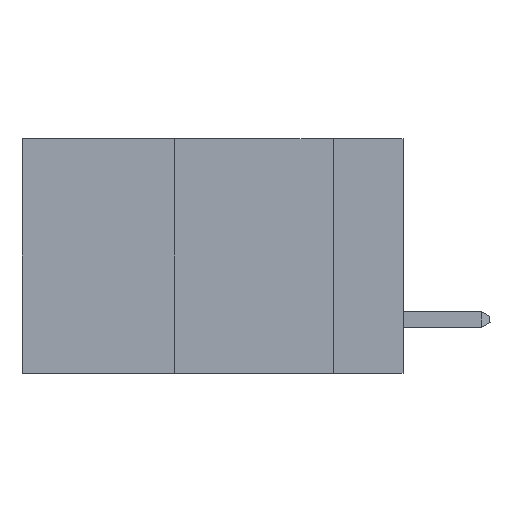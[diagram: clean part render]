
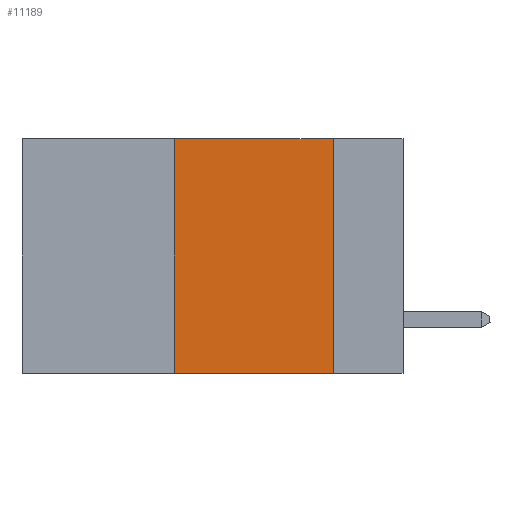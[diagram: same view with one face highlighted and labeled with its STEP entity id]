
A CAD part, left-side view. The second image highlights one B-rep face of the part: STEP entity #11189.
In plain terms, the highlighted planar face has unit normal (-1, 0, 0).
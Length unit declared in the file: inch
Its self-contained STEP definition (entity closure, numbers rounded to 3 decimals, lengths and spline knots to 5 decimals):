
#518 = VECTOR ( 'NONE', #11924, 39.37008 ) ;
#676 = ORIENTED_EDGE ( 'NONE', *, *, #15945, .F. ) ;
#3219 = DIRECTION ( 'NONE',  ( 0., 0., 1. ) ) ;
#4948 = VERTEX_POINT ( 'NONE', #10460 ) ;
#5170 = CARTESIAN_POINT ( 'NONE',  ( 0., 0.36, 0. ) ) ;
#6214 = CARTESIAN_POINT ( 'NONE',  ( 0., 0.6, 0. ) ) ;
#6275 = PLANE ( 'NONE',  #13305 ) ;
#6618 = VECTOR ( 'NONE', #9168, 39.37008 ) ;
#7361 = CARTESIAN_POINT ( 'NONE',  ( 0., 0.11, 0. ) ) ;
#7703 = DIRECTION ( 'NONE',  ( 0., 0., -1. ) ) ;
#7907 = ORIENTED_EDGE ( 'NONE', *, *, #16621, .F. ) ;
#9168 = DIRECTION ( 'NONE',  ( 0., -1., 0. ) ) ;
#9289 = VECTOR ( 'NONE', #3219, 39.37008 ) ;
#10460 = CARTESIAN_POINT ( 'NONE',  ( 0., 0.11, -0.37 ) ) ;
#11070 = ORIENTED_EDGE ( 'NONE', *, *, #15046, .F. ) ;
#11098 = LINE ( 'NONE', #15953, #6618 ) ;
#11189 = ADVANCED_FACE ( 'NONE', ( #14646 ), #6275, .F. ) ;
#11464 = DIRECTION ( 'NONE',  ( 0., 0., -1. ) ) ;
#11812 = LINE ( 'NONE', #14694, #518 ) ;
#11924 = DIRECTION ( 'NONE',  ( 0., -1., 0. ) ) ;
#13004 = VERTEX_POINT ( 'NONE', #16023 ) ;
#13062 = CARTESIAN_POINT ( 'NONE',  ( 0., 0.36, 0. ) ) ;
#13305 = AXIS2_PLACEMENT_3D ( 'NONE', #6214, #15879, #7703 ) ;
#13361 = VECTOR ( 'NONE', #11464, 39.37008 ) ;
#13809 = LINE ( 'NONE', #7361, #13361 ) ;
#14348 = EDGE_LOOP ( 'NONE', ( #11070, #7907, #676, #15606 ) ) ;
#14646 = FACE_OUTER_BOUND ( 'NONE', #14348, .T. ) ;
#14694 = CARTESIAN_POINT ( 'NONE',  ( 0., 0.6, 0. ) ) ;
#14949 = VERTEX_POINT ( 'NONE', #16719 ) ;
#15046 = EDGE_CURVE ( 'NONE', #14949, #4948, #13809, .T. ) ;
#15606 = ORIENTED_EDGE ( 'NONE', *, *, #17745, .T. ) ;
#15879 = DIRECTION ( 'NONE',  ( 1., 0., 0. ) ) ;
#15945 = EDGE_CURVE ( 'NONE', #13004, #16123, #16526, .T. ) ;
#15953 = CARTESIAN_POINT ( 'NONE',  ( 0., 0.6, -0.37 ) ) ;
#16023 = CARTESIAN_POINT ( 'NONE',  ( 0., 0.36, -0.37 ) ) ;
#16123 = VERTEX_POINT ( 'NONE', #5170 ) ;
#16526 = LINE ( 'NONE', #13062, #9289 ) ;
#16621 = EDGE_CURVE ( 'NONE', #16123, #14949, #11812, .T. ) ;
#16719 = CARTESIAN_POINT ( 'NONE',  ( 0., 0.11, 0. ) ) ;
#17745 = EDGE_CURVE ( 'NONE', #13004, #4948, #11098, .T. ) ;
